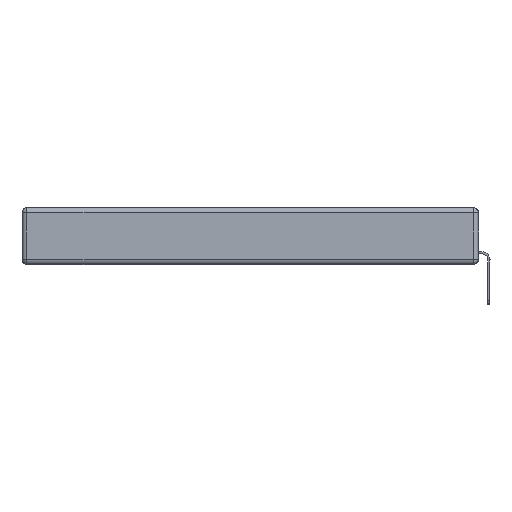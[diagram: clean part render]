
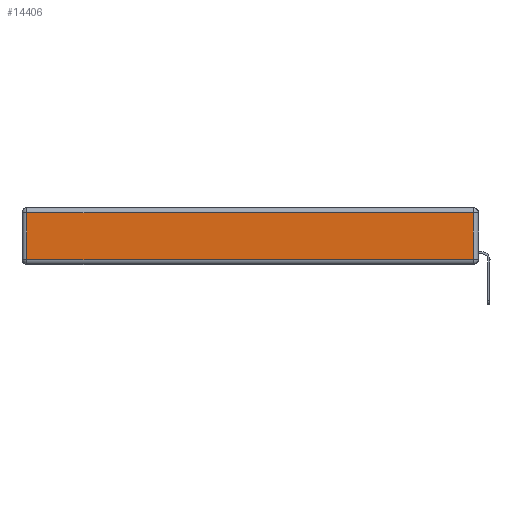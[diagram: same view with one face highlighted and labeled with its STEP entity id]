
A CAD part, left-side view. The second image highlights one B-rep face of the part: STEP entity #14406.
In plain terms, the highlighted planar face has unit normal (-1, 0, 0).
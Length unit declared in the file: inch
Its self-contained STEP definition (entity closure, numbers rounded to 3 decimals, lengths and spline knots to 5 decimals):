
#1173 = DIRECTION ( 'NONE',  ( 0., 0., 1. ) ) ;
#1254 = CARTESIAN_POINT ( 'NONE',  ( 0., 0., -0.313 ) ) ;
#2197 = VERTEX_POINT ( 'NONE', #7614 ) ;
#3136 = LINE ( 'NONE', #10389, #19978 ) ;
#4336 = CARTESIAN_POINT ( 'NONE',  ( 0., 0., -0.343 ) ) ;
#4359 = EDGE_CURVE ( 'NONE', #17736, #2197, #3136, .T. ) ;
#4448 = FACE_OUTER_BOUND ( 'NONE', #21186, .T. ) ;
#5620 = CARTESIAN_POINT ( 'NONE',  ( 0., 2.72, -0.03 ) ) ;
#6092 = ORIENTED_EDGE ( 'NONE', *, *, #17605, .T. ) ;
#6230 = DIRECTION ( 'NONE',  ( 0., 0., 1. ) ) ;
#7614 = CARTESIAN_POINT ( 'NONE',  ( 0., 2.72, -0.313 ) ) ;
#7889 = VECTOR ( 'NONE', #8382, 39.37008 ) ;
#8382 = DIRECTION ( 'NONE',  ( 0., -1., 0. ) ) ;
#10320 = LINE ( 'NONE', #17429, #23181 ) ;
#10389 = CARTESIAN_POINT ( 'NONE',  ( 0., 2.72, -0.343 ) ) ;
#11816 = PLANE ( 'NONE',  #22046 ) ;
#12185 = ORIENTED_EDGE ( 'NONE', *, *, #4359, .T. ) ;
#12616 = CARTESIAN_POINT ( 'NONE',  ( 0., 2.75, -0.03 ) ) ;
#12829 = DIRECTION ( 'NONE',  ( 0., 1., 0. ) ) ;
#13715 = DIRECTION ( 'NONE',  ( -1., 0., 0. ) ) ;
#14215 = CARTESIAN_POINT ( 'NONE',  ( 0., 0.03, -0.313 ) ) ;
#14378 = LINE ( 'NONE', #12616, #15250 ) ;
#14406 = ADVANCED_FACE ( 'NONE', ( #4448 ), #11816, .T. ) ;
#15170 = EDGE_CURVE ( 'NONE', #18878, #17736, #14378, .T. ) ;
#15250 = VECTOR ( 'NONE', #12829, 39.37008 ) ;
#17429 = CARTESIAN_POINT ( 'NONE',  ( 0., 0.03, -0.343 ) ) ;
#17605 = EDGE_CURVE ( 'NONE', #2197, #19045, #23205, .T. ) ;
#17736 = VERTEX_POINT ( 'NONE', #5620 ) ;
#17755 = ORIENTED_EDGE ( 'NONE', *, *, #22038, .T. ) ;
#18878 = VERTEX_POINT ( 'NONE', #21213 ) ;
#18925 = DIRECTION ( 'NONE',  ( 0., 0., -1. ) ) ;
#19045 = VERTEX_POINT ( 'NONE', #14215 ) ;
#19978 = VECTOR ( 'NONE', #18925, 39.37008 ) ;
#21186 = EDGE_LOOP ( 'NONE', ( #6092, #17755, #23293, #12185 ) ) ;
#21213 = CARTESIAN_POINT ( 'NONE',  ( 0., 0.03, -0.03 ) ) ;
#22038 = EDGE_CURVE ( 'NONE', #19045, #18878, #10320, .T. ) ;
#22046 = AXIS2_PLACEMENT_3D ( 'NONE', #4336, #13715, #6230 ) ;
#23181 = VECTOR ( 'NONE', #1173, 39.37008 ) ;
#23205 = LINE ( 'NONE', #1254, #7889 ) ;
#23293 = ORIENTED_EDGE ( 'NONE', *, *, #15170, .T. ) ;
